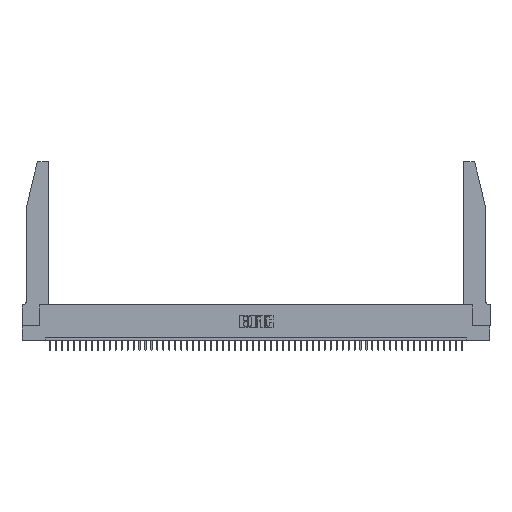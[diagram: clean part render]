
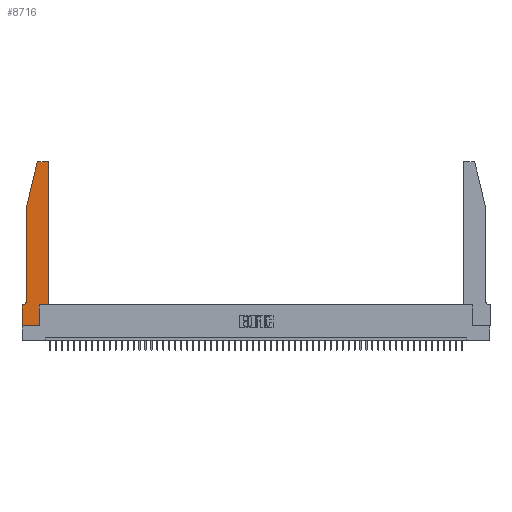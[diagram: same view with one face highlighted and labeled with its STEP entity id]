
A CAD part, top view. The second image highlights one B-rep face of the part: STEP entity #8716.
In plain terms, the highlighted planar face has unit normal (0, 0, 1).
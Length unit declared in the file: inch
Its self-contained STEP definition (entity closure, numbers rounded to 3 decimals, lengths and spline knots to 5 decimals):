
#663 = CARTESIAN_POINT ( 'NONE',  ( 0.0755, 0.35, 0.37 ) ) ;
#751 = VERTEX_POINT ( 'NONE', #46989 ) ;
#785 = DIRECTION ( 'NONE',  ( 0., -1., 0. ) ) ;
#1073 = LINE ( 'NONE', #4409, #48456 ) ;
#1526 = ORIENTED_EDGE ( 'NONE', *, *, #51130, .T. ) ;
#3024 = ORIENTED_EDGE ( 'NONE', *, *, #11935, .T. ) ;
#3292 = CARTESIAN_POINT ( 'NONE',  ( 0.0755, 2., 0.37 ) ) ;
#3325 = VECTOR ( 'NONE', #11096, 39.37008 ) ;
#4215 = CARTESIAN_POINT ( 'NONE',  ( 0.0055, 0.35, 0.37 ) ) ;
#4409 = CARTESIAN_POINT ( 'NONE',  ( 0., 0., 0.37 ) ) ;
#5017 = DIRECTION ( 'NONE',  ( 0., 0., -1. ) ) ;
#5401 = VERTEX_POINT ( 'NONE', #15436 ) ;
#7317 = CARTESIAN_POINT ( 'NONE',  ( 0.0755, 2., 0.37 ) ) ;
#8122 = DIRECTION ( 'NONE',  ( 0., 1., 0. ) ) ;
#8650 = CARTESIAN_POINT ( 'NONE',  ( 0.284, 2.72, 0.37 ) ) ;
#8716 = ADVANCED_FACE ( 'NONE', ( #36305 ), #18890, .T. ) ;
#9676 = DIRECTION ( 'NONE',  ( 1., 0., 0. ) ) ;
#10016 = CARTESIAN_POINT ( 'NONE',  ( 0.4505, 0.35, 0.37 ) ) ;
#11096 = DIRECTION ( 'NONE',  ( 0., -1., 0. ) ) ;
#11935 = EDGE_CURVE ( 'NONE', #48255, #5401, #30021, .T. ) ;
#12411 = CARTESIAN_POINT ( 'NONE',  ( 0.2605, 2.75, 0.37 ) ) ;
#12418 = VERTEX_POINT ( 'NONE', #19972 ) ;
#12771 = VECTOR ( 'NONE', #21155, 39.37008 ) ;
#13562 = CARTESIAN_POINT ( 'NONE',  ( 0.4205, 2.75, 0.37 ) ) ;
#14760 = CARTESIAN_POINT ( 'NONE',  ( 0.4505, 0.35, 0.37 ) ) ;
#15436 = CARTESIAN_POINT ( 'NONE',  ( 0.25487, 2.72718, 0.37 ) ) ;
#15719 = CIRCLE ( 'NONE', #17534, 0.03 ) ;
#15947 = ORIENTED_EDGE ( 'NONE', *, *, #31320, .T. ) ;
#17376 = DIRECTION ( 'NONE',  ( -1., 0., 0. ) ) ;
#17534 = AXIS2_PLACEMENT_3D ( 'NONE', #48400, #44433, #43904 ) ;
#18468 = EDGE_CURVE ( 'NONE', #19314, #21188, #20392, .T. ) ;
#18698 = DIRECTION ( 'NONE',  ( 1., 0., 0. ) ) ;
#18890 = PLANE ( 'NONE',  #35679 ) ;
#19314 = VERTEX_POINT ( 'NONE', #14760 ) ;
#19972 = CARTESIAN_POINT ( 'NONE',  ( 0.0755, 0.42, 0.37 ) ) ;
#20392 = LINE ( 'NONE', #10016, #22970 ) ;
#21155 = DIRECTION ( 'NONE',  ( -0.239, -0.971, 0. ) ) ;
#21188 = VERTEX_POINT ( 'NONE', #28242 ) ;
#21496 = DIRECTION ( 'NONE',  ( -1., 0., 0. ) ) ;
#22299 = ORIENTED_EDGE ( 'NONE', *, *, #42097, .T. ) ;
#22451 = EDGE_CURVE ( 'NONE', #28221, #48255, #24979, .T. ) ;
#22956 = CARTESIAN_POINT ( 'NONE',  ( 0.2865, 0., 0.37 ) ) ;
#22970 = VECTOR ( 'NONE', #39793, 39.37008 ) ;
#23104 = VERTEX_POINT ( 'NONE', #22956 ) ;
#23339 = VECTOR ( 'NONE', #9676, 39.37008 ) ;
#23399 = DIRECTION ( 'NONE',  ( 0., 0., 1. ) ) ;
#24135 = DIRECTION ( 'NONE',  ( -1., 0., 0. ) ) ;
#24979 = LINE ( 'NONE', #12411, #34708 ) ;
#25347 = CARTESIAN_POINT ( 'NONE',  ( 0.4505, 0.35, 0.37 ) ) ;
#25728 = EDGE_CURVE ( 'NONE', #27968, #23104, #45448, .T. ) ;
#26598 = ORIENTED_EDGE ( 'NONE', *, *, #27715, .T. ) ;
#27202 = DIRECTION ( 'NONE',  ( 0., 0., 1. ) ) ;
#27715 = EDGE_CURVE ( 'NONE', #751, #27968, #1073, .T. ) ;
#27847 = CARTESIAN_POINT ( 'NONE',  ( 0., 0., 0.37 ) ) ;
#27968 = VERTEX_POINT ( 'NONE', #27847 ) ;
#27983 = LINE ( 'NONE', #7317, #3325 ) ;
#28221 = VERTEX_POINT ( 'NONE', #13562 ) ;
#28242 = CARTESIAN_POINT ( 'NONE',  ( 0.4505, 2.72, 0.37 ) ) ;
#28558 = VECTOR ( 'NONE', #21496, 39.37008 ) ;
#28964 = DIRECTION ( 'NONE',  ( 1., 0., 0. ) ) ;
#29165 = DIRECTION ( 'NONE',  ( 1., 0., 0. ) ) ;
#29755 = ORIENTED_EDGE ( 'NONE', *, *, #22451, .T. ) ;
#29858 = CARTESIAN_POINT ( 'NONE',  ( 0.0055, 0.42, 0.37 ) ) ;
#29881 = CARTESIAN_POINT ( 'NONE',  ( 0.284, 2.75, 0.37 ) ) ;
#30021 = CIRCLE ( 'NONE', #37487, 0.03 ) ;
#30028 = VECTOR ( 'NONE', #29165, 39.37008 ) ;
#30190 = EDGE_CURVE ( 'NONE', #12418, #49998, #45645, .T. ) ;
#30495 = LINE ( 'NONE', #663, #28558 ) ;
#31320 = EDGE_CURVE ( 'NONE', #21188, #28221, #15719, .T. ) ;
#32821 = AXIS2_PLACEMENT_3D ( 'NONE', #29858, #5017, #17376 ) ;
#32981 = CARTESIAN_POINT ( 'NONE',  ( 0.2865, 0.35, 0.37 ) ) ;
#33312 = ORIENTED_EDGE ( 'NONE', *, *, #34250, .T. ) ;
#33337 = ORIENTED_EDGE ( 'NONE', *, *, #25728, .T. ) ;
#34250 = EDGE_CURVE ( 'NONE', #43739, #12418, #27983, .T. ) ;
#34516 = CARTESIAN_POINT ( 'NONE',  ( 0., 0., 0.37 ) ) ;
#34708 = VECTOR ( 'NONE', #24135, 39.37008 ) ;
#35328 = ORIENTED_EDGE ( 'NONE', *, *, #45163, .T. ) ;
#35679 = AXIS2_PLACEMENT_3D ( 'NONE', #48260, #23399, #18698 ) ;
#36305 = FACE_OUTER_BOUND ( 'NONE', #42705, .T. ) ;
#37214 = LINE ( 'NONE', #25347, #30028 ) ;
#37487 = AXIS2_PLACEMENT_3D ( 'NONE', #8650, #27202, #28964 ) ;
#37689 = ORIENTED_EDGE ( 'NONE', *, *, #30190, .T. ) ;
#38611 = CARTESIAN_POINT ( 'NONE',  ( 0.2865, 0.35, 0.37 ) ) ;
#39107 = ORIENTED_EDGE ( 'NONE', *, *, #46769, .T. ) ;
#39793 = DIRECTION ( 'NONE',  ( 0., 1., 0. ) ) ;
#41164 = VECTOR ( 'NONE', #8122, 39.37008 ) ;
#42097 = EDGE_CURVE ( 'NONE', #5401, #43739, #53698, .T. ) ;
#42636 = ORIENTED_EDGE ( 'NONE', *, *, #18468, .T. ) ;
#42705 = EDGE_LOOP ( 'NONE', ( #29755, #3024, #22299, #33312, #37689, #39107, #26598, #33337, #1526, #35328, #42636, #15947 ) ) ;
#43288 = VERTEX_POINT ( 'NONE', #38611 ) ;
#43739 = VERTEX_POINT ( 'NONE', #3292 ) ;
#43904 = DIRECTION ( 'NONE',  ( 1., 0., 0. ) ) ;
#44433 = DIRECTION ( 'NONE',  ( 0., 0., 1. ) ) ;
#45163 = EDGE_CURVE ( 'NONE', #43288, #19314, #37214, .T. ) ;
#45448 = LINE ( 'NONE', #34516, #23339 ) ;
#45645 = CIRCLE ( 'NONE', #32821, 0.07 ) ;
#46769 = EDGE_CURVE ( 'NONE', #49998, #751, #30495, .T. ) ;
#46989 = CARTESIAN_POINT ( 'NONE',  ( 0., 0.35, 0.37 ) ) ;
#48255 = VERTEX_POINT ( 'NONE', #29881 ) ;
#48260 = CARTESIAN_POINT ( 'NONE',  ( 0., 0.35, 0.37 ) ) ;
#48400 = CARTESIAN_POINT ( 'NONE',  ( 0.4205, 2.72, 0.37 ) ) ;
#48456 = VECTOR ( 'NONE', #785, 39.37008 ) ;
#49644 = CARTESIAN_POINT ( 'NONE',  ( 0.0755, 2., 0.37 ) ) ;
#49998 = VERTEX_POINT ( 'NONE', #4215 ) ;
#51130 = EDGE_CURVE ( 'NONE', #23104, #43288, #52156, .T. ) ;
#52156 = LINE ( 'NONE', #32981, #41164 ) ;
#53698 = LINE ( 'NONE', #49644, #12771 ) ;
